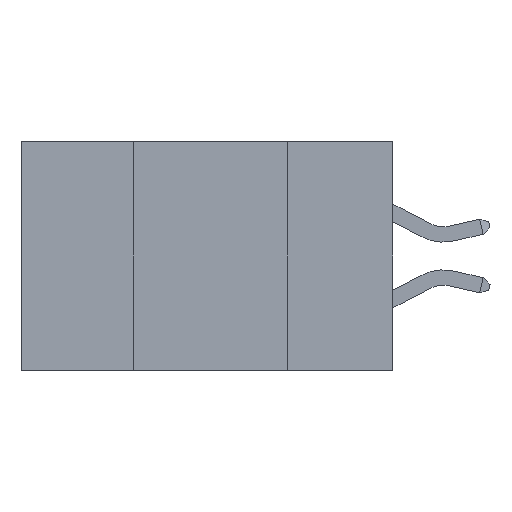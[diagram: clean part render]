
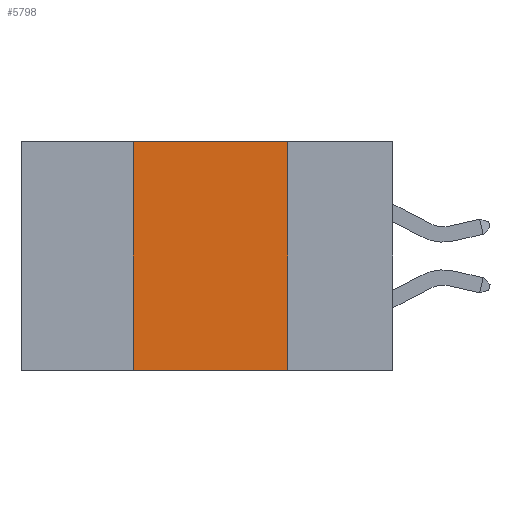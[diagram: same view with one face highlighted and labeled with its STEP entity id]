
A CAD part, left-side view. The second image highlights one B-rep face of the part: STEP entity #5798.
In plain terms, the highlighted planar face has unit normal (-1, 0, 0).
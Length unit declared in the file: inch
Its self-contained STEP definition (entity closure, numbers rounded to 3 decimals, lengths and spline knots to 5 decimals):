
#574 = DIRECTION ( 'NONE',  ( 0., -1., 0. ) ) ;
#1393 = EDGE_LOOP ( 'NONE', ( #13301, #24852, #22210, #6730 ) ) ;
#1628 = DIRECTION ( 'NONE',  ( 0., 0., -1. ) ) ;
#1913 = LINE ( 'NONE', #25388, #22761 ) ;
#2573 = CARTESIAN_POINT ( 'NONE',  ( 0., 0.6, 0. ) ) ;
#4268 = VECTOR ( 'NONE', #19904, 39.37008 ) ;
#4525 = CARTESIAN_POINT ( 'NONE',  ( 0., 0.17, -0.37 ) ) ;
#4606 = EDGE_CURVE ( 'NONE', #17212, #13042, #10895, .T. ) ;
#5311 = VECTOR ( 'NONE', #22024, 39.37008 ) ;
#5469 = AXIS2_PLACEMENT_3D ( 'NONE', #13165, #5541, #1628 ) ;
#5482 = VECTOR ( 'NONE', #574, 39.37008 ) ;
#5541 = DIRECTION ( 'NONE',  ( 1., 0., 0. ) ) ;
#5798 = ADVANCED_FACE ( 'NONE', ( #10499 ), #21164, .F. ) ;
#6178 = CARTESIAN_POINT ( 'NONE',  ( 0., 0.17, 0. ) ) ;
#6730 = ORIENTED_EDGE ( 'NONE', *, *, #23420, .T. ) ;
#6961 = DIRECTION ( 'NONE',  ( 0., 0., -1. ) ) ;
#7674 = EDGE_CURVE ( 'NONE', #25657, #17212, #9704, .T. ) ;
#9704 = LINE ( 'NONE', #14180, #4268 ) ;
#10499 = FACE_OUTER_BOUND ( 'NONE', #1393, .T. ) ;
#10856 = EDGE_CURVE ( 'NONE', #13042, #26130, #1913, .T. ) ;
#10895 = LINE ( 'NONE', #2573, #5482 ) ;
#12898 = LINE ( 'NONE', #15162, #5311 ) ;
#13042 = VERTEX_POINT ( 'NONE', #6178 ) ;
#13165 = CARTESIAN_POINT ( 'NONE',  ( 0., 0.6, 0. ) ) ;
#13170 = CARTESIAN_POINT ( 'NONE',  ( 0., 0.42, 0. ) ) ;
#13301 = ORIENTED_EDGE ( 'NONE', *, *, #10856, .F. ) ;
#14180 = CARTESIAN_POINT ( 'NONE',  ( 0., 0.42, 0. ) ) ;
#15162 = CARTESIAN_POINT ( 'NONE',  ( 0., 0.6, -0.37 ) ) ;
#17212 = VERTEX_POINT ( 'NONE', #13170 ) ;
#19904 = DIRECTION ( 'NONE',  ( 0., 0., 1. ) ) ;
#21164 = PLANE ( 'NONE',  #5469 ) ;
#22024 = DIRECTION ( 'NONE',  ( 0., -1., 0. ) ) ;
#22210 = ORIENTED_EDGE ( 'NONE', *, *, #7674, .F. ) ;
#22761 = VECTOR ( 'NONE', #6961, 39.37008 ) ;
#23420 = EDGE_CURVE ( 'NONE', #25657, #26130, #12898, .T. ) ;
#24546 = CARTESIAN_POINT ( 'NONE',  ( 0., 0.42, -0.37 ) ) ;
#24852 = ORIENTED_EDGE ( 'NONE', *, *, #4606, .F. ) ;
#25388 = CARTESIAN_POINT ( 'NONE',  ( 0., 0.17, 0. ) ) ;
#25657 = VERTEX_POINT ( 'NONE', #24546 ) ;
#26130 = VERTEX_POINT ( 'NONE', #4525 ) ;
